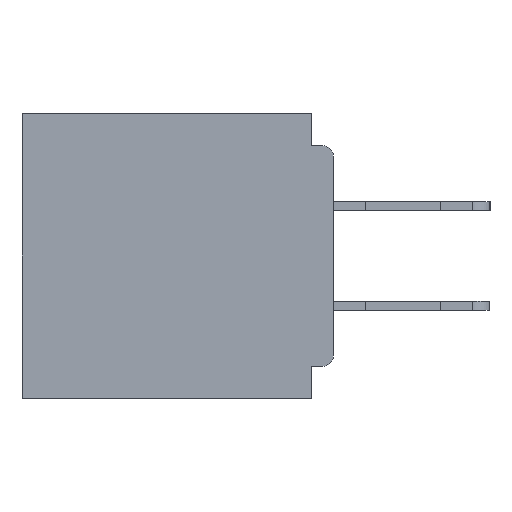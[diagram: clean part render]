
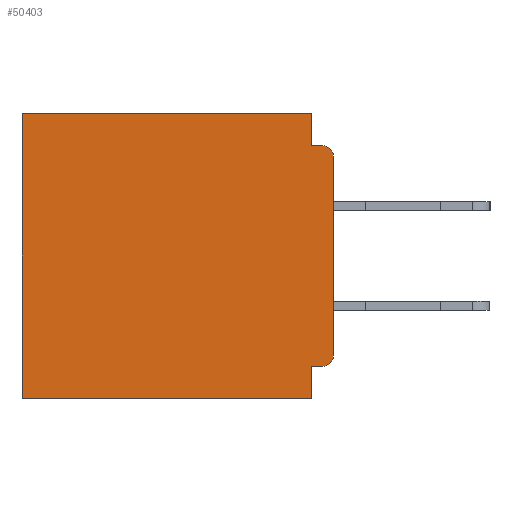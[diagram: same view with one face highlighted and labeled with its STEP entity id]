
A CAD part, left-side view. The second image highlights one B-rep face of the part: STEP entity #50403.
In plain terms, the highlighted planar face has unit normal (-1, 0, 0).
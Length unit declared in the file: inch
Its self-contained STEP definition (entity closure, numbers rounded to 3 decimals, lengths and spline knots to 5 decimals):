
#254 = CARTESIAN_POINT ( 'NONE',  ( 0.3, 0., -0.4 ) ) ;
#1414 = VECTOR ( 'NONE', #4642, 39.37008 ) ;
#1479 = DIRECTION ( 'NONE',  ( 0., 0., -1. ) ) ;
#2795 = VERTEX_POINT ( 'NONE', #30238 ) ;
#2801 = LINE ( 'NONE', #254, #1414 ) ;
#2998 = ORIENTED_EDGE ( 'NONE', *, *, #54291, .F. ) ;
#3319 = DIRECTION ( 'NONE',  ( 0., 0., -1. ) ) ;
#3463 = AXIS2_PLACEMENT_3D ( 'NONE', #9951, #40248, #14277 ) ;
#3822 = CARTESIAN_POINT ( 'NONE',  ( 0.3, 0.031, 0. ) ) ;
#4390 = AXIS2_PLACEMENT_3D ( 'NONE', #53202, #27394, #1479 ) ;
#4642 = DIRECTION ( 'NONE',  ( 0., 0., -1. ) ) ;
#5685 = VERTEX_POINT ( 'NONE', #3822 ) ;
#7099 = CARTESIAN_POINT ( 'NONE',  ( 0.3, 0.015, -0.045 ) ) ;
#7696 = CARTESIAN_POINT ( 'NONE',  ( 0.3, 0., -0.045 ) ) ;
#8029 = EDGE_CURVE ( 'NONE', #44692, #28207, #39422, .T. ) ;
#8588 = EDGE_CURVE ( 'NONE', #23889, #40765, #49320, .T. ) ;
#9750 = LINE ( 'NONE', #49410, #31446 ) ;
#9951 = CARTESIAN_POINT ( 'NONE',  ( 0.3, 0.015, -0.06 ) ) ;
#10200 = VERTEX_POINT ( 'NONE', #53402 ) ;
#10463 = CARTESIAN_POINT ( 'NONE',  ( 0.3, 0., -0.34 ) ) ;
#11774 = LINE ( 'NONE', #7696, #33481 ) ;
#12021 = DIRECTION ( 'NONE',  ( 0., -1., 0. ) ) ;
#14277 = DIRECTION ( 'NONE',  ( 0., 0., -1. ) ) ;
#16134 = PLANE ( 'NONE',  #35488 ) ;
#16188 = CARTESIAN_POINT ( 'NONE',  ( 0.3, 0.031, -0.4 ) ) ;
#16874 = VERTEX_POINT ( 'NONE', #50065 ) ;
#17193 = VECTOR ( 'NONE', #48826, 39.37008 ) ;
#18419 = ORIENTED_EDGE ( 'NONE', *, *, #8029, .T. ) ;
#18986 = CARTESIAN_POINT ( 'NONE',  ( 0.3, 0.437, -0.4 ) ) ;
#19749 = ORIENTED_EDGE ( 'NONE', *, *, #40639, .F. ) ;
#20599 = LINE ( 'NONE', #40265, #42311 ) ;
#21318 = VERTEX_POINT ( 'NONE', #7099 ) ;
#21368 = EDGE_CURVE ( 'NONE', #44692, #2795, #34366, .T. ) ;
#22574 = VERTEX_POINT ( 'NONE', #16188 ) ;
#23192 = CARTESIAN_POINT ( 'NONE',  ( 0.3, 0.015, -0.355 ) ) ;
#23889 = VERTEX_POINT ( 'NONE', #51090 ) ;
#24537 = ORIENTED_EDGE ( 'NONE', *, *, #51996, .T. ) ;
#25382 = EDGE_CURVE ( 'NONE', #10200, #21318, #55807, .T. ) ;
#25914 = ORIENTED_EDGE ( 'NONE', *, *, #8588, .T. ) ;
#27260 = EDGE_LOOP ( 'NONE', ( #47489, #53552, #52225, #19749, #24537, #25914, #46201, #2998, #53603, #18419 ) ) ;
#27387 = LINE ( 'NONE', #35636, #17193 ) ;
#27394 = DIRECTION ( 'NONE',  ( -1., 0., 0. ) ) ;
#28207 = VERTEX_POINT ( 'NONE', #10463 ) ;
#29227 = DIRECTION ( 'NONE',  ( 1., 0., 0. ) ) ;
#29456 = EDGE_CURVE ( 'NONE', #22574, #40765, #27387, .T. ) ;
#30238 = CARTESIAN_POINT ( 'NONE',  ( 0.3, 0.031, -0.355 ) ) ;
#30483 = CARTESIAN_POINT ( 'NONE',  ( 0.3, 0.031, 0. ) ) ;
#31446 = VECTOR ( 'NONE', #53731, 39.37008 ) ;
#33481 = VECTOR ( 'NONE', #12021, 39.37008 ) ;
#34366 = LINE ( 'NONE', #46378, #55881 ) ;
#34657 = DIRECTION ( 'NONE',  ( 0., 0., -1. ) ) ;
#35488 = AXIS2_PLACEMENT_3D ( 'NONE', #55023, #29227, #3319 ) ;
#35636 = CARTESIAN_POINT ( 'NONE',  ( 0.3, 0., -0.4 ) ) ;
#36655 = EDGE_CURVE ( 'NONE', #10200, #28207, #2801, .T. ) ;
#38221 = VECTOR ( 'NONE', #34657, 39.37008 ) ;
#39422 = CIRCLE ( 'NONE', #4390, 0.015 ) ;
#39562 = LINE ( 'NONE', #30483, #38221 ) ;
#40248 = DIRECTION ( 'NONE',  ( -1., 0., 0. ) ) ;
#40265 = CARTESIAN_POINT ( 'NONE',  ( 0.3, 0.031, -0.4 ) ) ;
#40639 = EDGE_CURVE ( 'NONE', #5685, #16874, #39562, .T. ) ;
#40765 = VERTEX_POINT ( 'NONE', #18986 ) ;
#42311 = VECTOR ( 'NONE', #44558, 39.37008 ) ;
#44558 = DIRECTION ( 'NONE',  ( 0., 0., -1. ) ) ;
#44692 = VERTEX_POINT ( 'NONE', #23192 ) ;
#46201 = ORIENTED_EDGE ( 'NONE', *, *, #29456, .F. ) ;
#46277 = DIRECTION ( 'NONE',  ( 0., 0., -1. ) ) ;
#46378 = CARTESIAN_POINT ( 'NONE',  ( 0.3, 0., -0.355 ) ) ;
#47489 = ORIENTED_EDGE ( 'NONE', *, *, #36655, .F. ) ;
#47984 = VECTOR ( 'NONE', #46277, 39.37008 ) ;
#48111 = CARTESIAN_POINT ( 'NONE',  ( 0.3, 0.437, -0.4 ) ) ;
#48826 = DIRECTION ( 'NONE',  ( 0., 1., 0. ) ) ;
#49320 = LINE ( 'NONE', #48111, #47984 ) ;
#49410 = CARTESIAN_POINT ( 'NONE',  ( 0.3, 0., 0. ) ) ;
#50065 = CARTESIAN_POINT ( 'NONE',  ( 0.3, 0.031, -0.045 ) ) ;
#50403 = ADVANCED_FACE ( 'NONE', ( #55777 ), #16134, .F. ) ;
#50693 = DIRECTION ( 'NONE',  ( 0., 1., 0. ) ) ;
#51090 = CARTESIAN_POINT ( 'NONE',  ( 0.3, 0.437, 0. ) ) ;
#51996 = EDGE_CURVE ( 'NONE', #5685, #23889, #9750, .T. ) ;
#52159 = EDGE_CURVE ( 'NONE', #16874, #21318, #11774, .T. ) ;
#52225 = ORIENTED_EDGE ( 'NONE', *, *, #52159, .F. ) ;
#53202 = CARTESIAN_POINT ( 'NONE',  ( 0.3, 0.015, -0.34 ) ) ;
#53402 = CARTESIAN_POINT ( 'NONE',  ( 0.3, 0., -0.06 ) ) ;
#53552 = ORIENTED_EDGE ( 'NONE', *, *, #25382, .T. ) ;
#53603 = ORIENTED_EDGE ( 'NONE', *, *, #21368, .F. ) ;
#53731 = DIRECTION ( 'NONE',  ( 0., 1., 0. ) ) ;
#54291 = EDGE_CURVE ( 'NONE', #2795, #22574, #20599, .T. ) ;
#55023 = CARTESIAN_POINT ( 'NONE',  ( 0.3, 0., -0.4 ) ) ;
#55777 = FACE_OUTER_BOUND ( 'NONE', #27260, .T. ) ;
#55807 = CIRCLE ( 'NONE', #3463, 0.015 ) ;
#55881 = VECTOR ( 'NONE', #50693, 39.37008 ) ;
